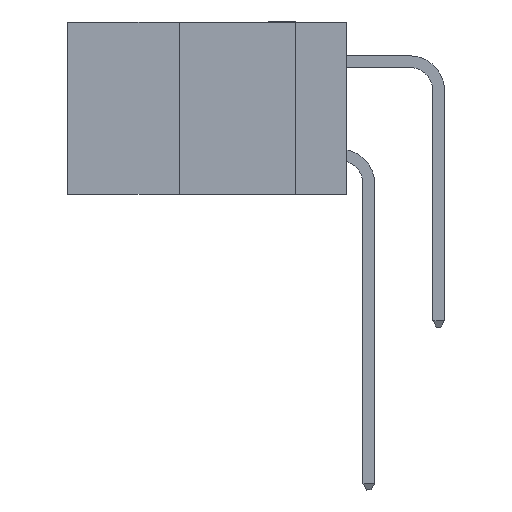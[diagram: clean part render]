
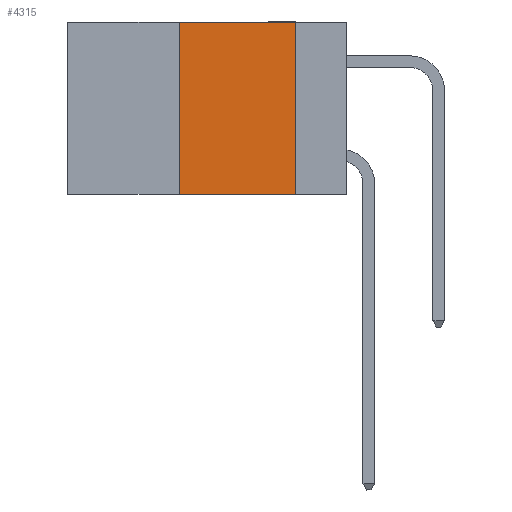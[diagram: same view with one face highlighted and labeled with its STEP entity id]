
A CAD part, left-side view. The second image highlights one B-rep face of the part: STEP entity #4315.
In plain terms, the highlighted planar face has unit normal (-1, 0, 0).
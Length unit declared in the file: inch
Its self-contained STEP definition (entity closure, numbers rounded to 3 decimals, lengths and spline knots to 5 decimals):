
#445 = LINE ( 'NONE', #5975, #1645 ) ;
#1466 = FACE_OUTER_BOUND ( 'NONE', #14757, .T. ) ;
#1645 = VECTOR ( 'NONE', #14944, 39.37008 ) ;
#2670 = VERTEX_POINT ( 'NONE', #15793 ) ;
#4072 = DIRECTION ( 'NONE',  ( 0., 0., -1. ) ) ;
#4263 = LINE ( 'NONE', #14110, #13466 ) ;
#4315 = ADVANCED_FACE ( 'NONE', ( #1466 ), #15662, .F. ) ;
#4442 = LINE ( 'NONE', #9544, #13647 ) ;
#4547 = EDGE_CURVE ( 'NONE', #16046, #9885, #4263, .T. ) ;
#4984 = AXIS2_PLACEMENT_3D ( 'NONE', #5585, #5477, #4072 ) ;
#5477 = DIRECTION ( 'NONE',  ( 1., 0., 0. ) ) ;
#5585 = CARTESIAN_POINT ( 'NONE',  ( 0., 0.6, 0. ) ) ;
#5975 = CARTESIAN_POINT ( 'NONE',  ( 0., 0.36, 0. ) ) ;
#5999 = ORIENTED_EDGE ( 'NONE', *, *, #6023, .F. ) ;
#6023 = EDGE_CURVE ( 'NONE', #7644, #16046, #4442, .T. ) ;
#7644 = VERTEX_POINT ( 'NONE', #9428 ) ;
#8401 = LINE ( 'NONE', #15168, #14201 ) ;
#8879 = ORIENTED_EDGE ( 'NONE', *, *, #13559, .F. ) ;
#9428 = CARTESIAN_POINT ( 'NONE',  ( 0., 0.36, 0. ) ) ;
#9544 = CARTESIAN_POINT ( 'NONE',  ( 0., 0.6, 0. ) ) ;
#9885 = VERTEX_POINT ( 'NONE', #14238 ) ;
#10373 = DIRECTION ( 'NONE',  ( 0., 0., -1. ) ) ;
#11342 = EDGE_CURVE ( 'NONE', #2670, #9885, #8401, .T. ) ;
#11959 = ORIENTED_EDGE ( 'NONE', *, *, #11342, .T. ) ;
#13466 = VECTOR ( 'NONE', #10373, 39.37008 ) ;
#13559 = EDGE_CURVE ( 'NONE', #2670, #7644, #445, .T. ) ;
#13647 = VECTOR ( 'NONE', #13738, 39.37008 ) ;
#13738 = DIRECTION ( 'NONE',  ( 0., -1., 0. ) ) ;
#13932 = DIRECTION ( 'NONE',  ( 0., -1., 0. ) ) ;
#14110 = CARTESIAN_POINT ( 'NONE',  ( 0., 0.11, 0. ) ) ;
#14201 = VECTOR ( 'NONE', #13932, 39.37008 ) ;
#14238 = CARTESIAN_POINT ( 'NONE',  ( 0., 0.11, -0.37 ) ) ;
#14757 = EDGE_LOOP ( 'NONE', ( #16250, #5999, #8879, #11959 ) ) ;
#14944 = DIRECTION ( 'NONE',  ( 0., 0., 1. ) ) ;
#15168 = CARTESIAN_POINT ( 'NONE',  ( 0., 0.6, -0.37 ) ) ;
#15263 = CARTESIAN_POINT ( 'NONE',  ( 0., 0.11, 0. ) ) ;
#15662 = PLANE ( 'NONE',  #4984 ) ;
#15793 = CARTESIAN_POINT ( 'NONE',  ( 0., 0.36, -0.37 ) ) ;
#16046 = VERTEX_POINT ( 'NONE', #15263 ) ;
#16250 = ORIENTED_EDGE ( 'NONE', *, *, #4547, .F. ) ;
